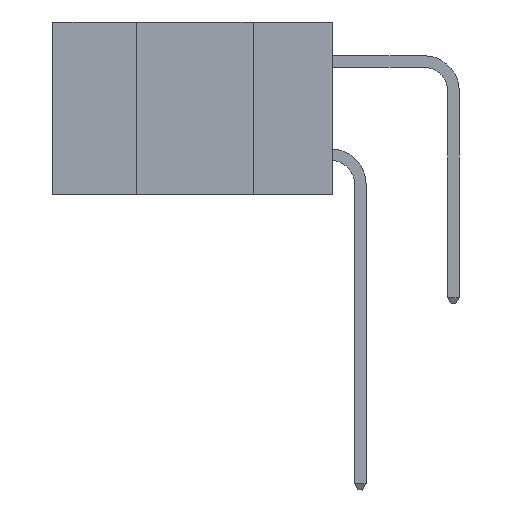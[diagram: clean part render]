
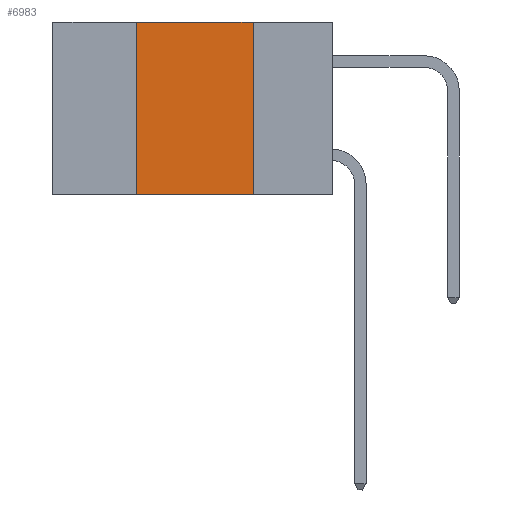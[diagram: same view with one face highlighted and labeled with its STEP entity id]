
A CAD part, left-side view. The second image highlights one B-rep face of the part: STEP entity #6983.
In plain terms, the highlighted planar face has unit normal (-1, 0, 0).
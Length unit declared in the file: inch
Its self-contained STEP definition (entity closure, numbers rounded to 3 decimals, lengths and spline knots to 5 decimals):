
#102 = CARTESIAN_POINT ( 'NONE',  ( 0., 0.17, 0. ) ) ;
#327 = VECTOR ( 'NONE', #11246, 39.37008 ) ;
#1022 = EDGE_CURVE ( 'NONE', #24189, #14555, #1703, .T. ) ;
#1703 = LINE ( 'NONE', #7167, #4813 ) ;
#2092 = CARTESIAN_POINT ( 'NONE',  ( 0., 0.6, 0. ) ) ;
#2323 = EDGE_LOOP ( 'NONE', ( #18682, #3417, #22155, #4350 ) ) ;
#3107 = LINE ( 'NONE', #22806, #327 ) ;
#3417 = ORIENTED_EDGE ( 'NONE', *, *, #3774, .F. ) ;
#3774 = EDGE_CURVE ( 'NONE', #7903, #15349, #12449, .T. ) ;
#4350 = ORIENTED_EDGE ( 'NONE', *, *, #1022, .T. ) ;
#4813 = VECTOR ( 'NONE', #25343, 39.37008 ) ;
#6983 = ADVANCED_FACE ( 'NONE', ( #25394 ), #13717, .F. ) ;
#7076 = VECTOR ( 'NONE', #21345, 39.37008 ) ;
#7167 = CARTESIAN_POINT ( 'NONE',  ( 0., 0.6, -0.37 ) ) ;
#7396 = CARTESIAN_POINT ( 'NONE',  ( 0., 0.42, 0. ) ) ;
#7903 = VERTEX_POINT ( 'NONE', #7396 ) ;
#8104 = DIRECTION ( 'NONE',  ( 0., 0., -1. ) ) ;
#8530 = DIRECTION ( 'NONE',  ( 0., -1., 0. ) ) ;
#9839 = AXIS2_PLACEMENT_3D ( 'NONE', #2092, #17627, #8104 ) ;
#11233 = EDGE_CURVE ( 'NONE', #15349, #14555, #17779, .T. ) ;
#11246 = DIRECTION ( 'NONE',  ( 0., 0., 1. ) ) ;
#12449 = LINE ( 'NONE', #18126, #16401 ) ;
#13717 = PLANE ( 'NONE',  #9839 ) ;
#14555 = VERTEX_POINT ( 'NONE', #15004 ) ;
#14790 = EDGE_CURVE ( 'NONE', #24189, #7903, #3107, .T. ) ;
#15004 = CARTESIAN_POINT ( 'NONE',  ( 0., 0.17, -0.37 ) ) ;
#15349 = VERTEX_POINT ( 'NONE', #102 ) ;
#16401 = VECTOR ( 'NONE', #8530, 39.37008 ) ;
#17231 = CARTESIAN_POINT ( 'NONE',  ( 0., 0.42, -0.37 ) ) ;
#17627 = DIRECTION ( 'NONE',  ( 1., 0., 0. ) ) ;
#17779 = LINE ( 'NONE', #23298, #7076 ) ;
#18126 = CARTESIAN_POINT ( 'NONE',  ( 0., 0.6, 0. ) ) ;
#18682 = ORIENTED_EDGE ( 'NONE', *, *, #11233, .F. ) ;
#21345 = DIRECTION ( 'NONE',  ( 0., 0., -1. ) ) ;
#22155 = ORIENTED_EDGE ( 'NONE', *, *, #14790, .F. ) ;
#22806 = CARTESIAN_POINT ( 'NONE',  ( 0., 0.42, 0. ) ) ;
#23298 = CARTESIAN_POINT ( 'NONE',  ( 0., 0.17, 0. ) ) ;
#24189 = VERTEX_POINT ( 'NONE', #17231 ) ;
#25343 = DIRECTION ( 'NONE',  ( 0., -1., 0. ) ) ;
#25394 = FACE_OUTER_BOUND ( 'NONE', #2323, .T. ) ;
